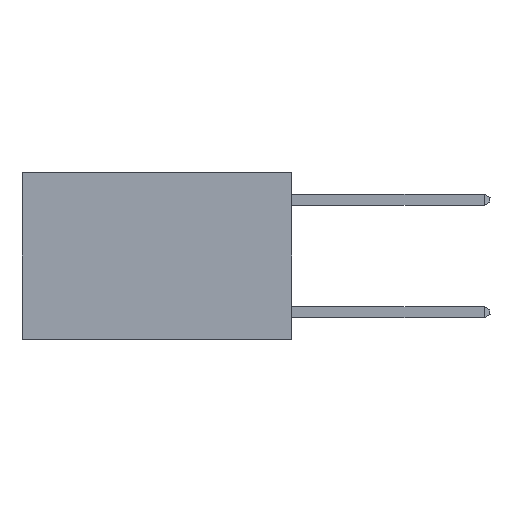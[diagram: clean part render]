
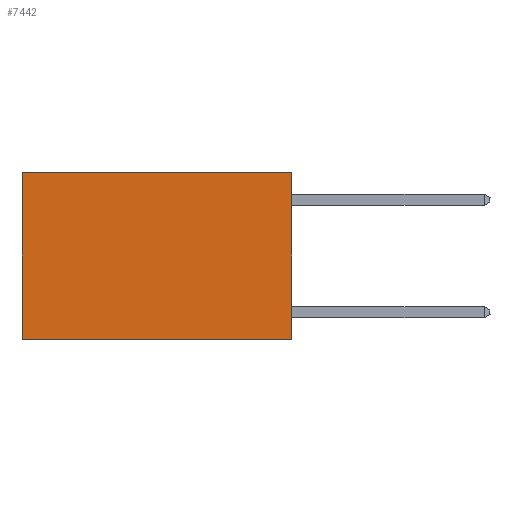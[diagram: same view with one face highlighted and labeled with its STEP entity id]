
A CAD part, left-side view. The second image highlights one B-rep face of the part: STEP entity #7442.
In plain terms, the highlighted planar face has unit normal (-1, 0, 0).
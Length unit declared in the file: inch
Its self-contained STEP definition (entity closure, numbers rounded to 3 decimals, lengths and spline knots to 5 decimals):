
#743 = DIRECTION ( 'NONE',  ( 0., 0., -1. ) ) ;
#748 = CARTESIAN_POINT ( 'NONE',  ( 0.2625, 0., 0. ) ) ;
#1190 = CARTESIAN_POINT ( 'NONE',  ( 0.2625, 0., 0. ) ) ;
#1563 = ORIENTED_EDGE ( 'NONE', *, *, #17300, .T. ) ;
#3081 = CARTESIAN_POINT ( 'NONE',  ( 0.2625, 0., -0.37 ) ) ;
#3451 = ORIENTED_EDGE ( 'NONE', *, *, #7697, .F. ) ;
#3533 = ORIENTED_EDGE ( 'NONE', *, *, #11769, .T. ) ;
#3917 = DIRECTION ( 'NONE',  ( 0., 0., -1. ) ) ;
#4385 = CARTESIAN_POINT ( 'NONE',  ( 0.2625, 0.6, -0.37 ) ) ;
#4523 = DIRECTION ( 'NONE',  ( 0., 1., 0. ) ) ;
#4549 = PLANE ( 'NONE',  #9067 ) ;
#4575 = EDGE_CURVE ( 'NONE', #5510, #6868, #13046, .T. ) ;
#4677 = VECTOR ( 'NONE', #4523, 39.37008 ) ;
#5510 = VERTEX_POINT ( 'NONE', #18855 ) ;
#6868 = VERTEX_POINT ( 'NONE', #4385 ) ;
#7442 = ADVANCED_FACE ( 'NONE', ( #14390 ), #4549, .F. ) ;
#7697 = EDGE_CURVE ( 'NONE', #17396, #5510, #8292, .T. ) ;
#8292 = LINE ( 'NONE', #11263, #15603 ) ;
#8732 = CARTESIAN_POINT ( 'NONE',  ( 0.2625, 0.6, 0. ) ) ;
#9067 = AXIS2_PLACEMENT_3D ( 'NONE', #13074, #12978, #14595 ) ;
#10102 = VECTOR ( 'NONE', #3917, 39.37008 ) ;
#11263 = CARTESIAN_POINT ( 'NONE',  ( 0.2625, 0., 0. ) ) ;
#11769 = EDGE_CURVE ( 'NONE', #17396, #17044, #15641, .T. ) ;
#12540 = LINE ( 'NONE', #14048, #10102 ) ;
#12978 = DIRECTION ( 'NONE',  ( 1., 0., 0. ) ) ;
#13046 = LINE ( 'NONE', #3081, #4677 ) ;
#13074 = CARTESIAN_POINT ( 'NONE',  ( 0.2625, 0., 0. ) ) ;
#14048 = CARTESIAN_POINT ( 'NONE',  ( 0.2625, 0.6, 0. ) ) ;
#14390 = FACE_OUTER_BOUND ( 'NONE', #15224, .T. ) ;
#14595 = DIRECTION ( 'NONE',  ( 0., 0., -1. ) ) ;
#15224 = EDGE_LOOP ( 'NONE', ( #1563, #17367, #3451, #3533 ) ) ;
#15603 = VECTOR ( 'NONE', #743, 39.37008 ) ;
#15641 = LINE ( 'NONE', #1190, #17593 ) ;
#15822 = DIRECTION ( 'NONE',  ( 0., 1., 0. ) ) ;
#17044 = VERTEX_POINT ( 'NONE', #8732 ) ;
#17300 = EDGE_CURVE ( 'NONE', #17044, #6868, #12540, .T. ) ;
#17367 = ORIENTED_EDGE ( 'NONE', *, *, #4575, .F. ) ;
#17396 = VERTEX_POINT ( 'NONE', #748 ) ;
#17593 = VECTOR ( 'NONE', #15822, 39.37008 ) ;
#18855 = CARTESIAN_POINT ( 'NONE',  ( 0.2625, 0., -0.37 ) ) ;
